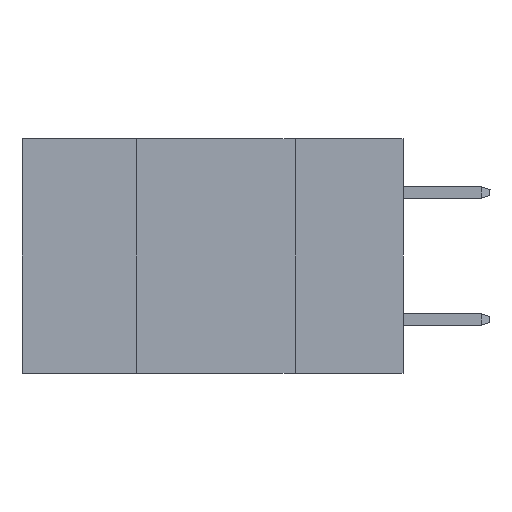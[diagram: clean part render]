
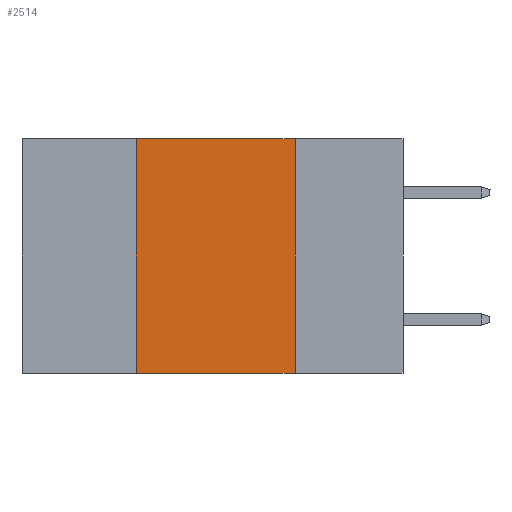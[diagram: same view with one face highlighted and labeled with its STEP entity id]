
A CAD part, left-side view. The second image highlights one B-rep face of the part: STEP entity #2514.
In plain terms, the highlighted planar face has unit normal (-1, 0, 0).
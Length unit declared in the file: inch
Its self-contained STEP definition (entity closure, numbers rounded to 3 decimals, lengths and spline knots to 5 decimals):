
#881 = FACE_OUTER_BOUND ( 'NONE', #6865, .T. ) ;
#942 = ORIENTED_EDGE ( 'NONE', *, *, #14671, .F. ) ;
#996 = LINE ( 'NONE', #6029, #6727 ) ;
#1439 = LINE ( 'NONE', #11648, #3242 ) ;
#2383 = DIRECTION ( 'NONE',  ( 0., 0., -1. ) ) ;
#2514 = ADVANCED_FACE ( 'NONE', ( #881 ), #5914, .F. ) ;
#3242 = VECTOR ( 'NONE', #11571, 39.37008 ) ;
#3357 = VECTOR ( 'NONE', #10164, 39.37008 ) ;
#4072 = VECTOR ( 'NONE', #12290, 39.37008 ) ;
#5055 = ORIENTED_EDGE ( 'NONE', *, *, #10624, .T. ) ;
#5520 = CARTESIAN_POINT ( 'NONE',  ( 0., 0.17, 0. ) ) ;
#5914 = PLANE ( 'NONE',  #9067 ) ;
#6029 = CARTESIAN_POINT ( 'NONE',  ( 0., 0.6, 0. ) ) ;
#6090 = EDGE_CURVE ( 'NONE', #12799, #13489, #13793, .T. ) ;
#6727 = VECTOR ( 'NONE', #11216, 39.37008 ) ;
#6865 = EDGE_LOOP ( 'NONE', ( #7540, #942, #14076, #5055 ) ) ;
#7318 = CARTESIAN_POINT ( 'NONE',  ( 0., 0.6, 0. ) ) ;
#7540 = ORIENTED_EDGE ( 'NONE', *, *, #6090, .F. ) ;
#8835 = CARTESIAN_POINT ( 'NONE',  ( 0., 0.42, 0. ) ) ;
#9067 = AXIS2_PLACEMENT_3D ( 'NONE', #7318, #11427, #2383 ) ;
#9722 = LINE ( 'NONE', #13516, #4072 ) ;
#10164 = DIRECTION ( 'NONE',  ( 0., 0., -1. ) ) ;
#10297 = EDGE_CURVE ( 'NONE', #10524, #15945, #1439, .T. ) ;
#10524 = VERTEX_POINT ( 'NONE', #14586 ) ;
#10624 = EDGE_CURVE ( 'NONE', #10524, #13489, #9722, .T. ) ;
#11216 = DIRECTION ( 'NONE',  ( 0., -1., 0. ) ) ;
#11427 = DIRECTION ( 'NONE',  ( 1., 0., 0. ) ) ;
#11549 = CARTESIAN_POINT ( 'NONE',  ( 0., 0.17, -0.37 ) ) ;
#11571 = DIRECTION ( 'NONE',  ( 0., 0., 1. ) ) ;
#11648 = CARTESIAN_POINT ( 'NONE',  ( 0., 0.42, 0. ) ) ;
#12290 = DIRECTION ( 'NONE',  ( 0., -1., 0. ) ) ;
#12799 = VERTEX_POINT ( 'NONE', #5520 ) ;
#13489 = VERTEX_POINT ( 'NONE', #11549 ) ;
#13516 = CARTESIAN_POINT ( 'NONE',  ( 0., 0.6, -0.37 ) ) ;
#13793 = LINE ( 'NONE', #13959, #3357 ) ;
#13959 = CARTESIAN_POINT ( 'NONE',  ( 0., 0.17, 0. ) ) ;
#14076 = ORIENTED_EDGE ( 'NONE', *, *, #10297, .F. ) ;
#14586 = CARTESIAN_POINT ( 'NONE',  ( 0., 0.42, -0.37 ) ) ;
#14671 = EDGE_CURVE ( 'NONE', #15945, #12799, #996, .T. ) ;
#15945 = VERTEX_POINT ( 'NONE', #8835 ) ;
